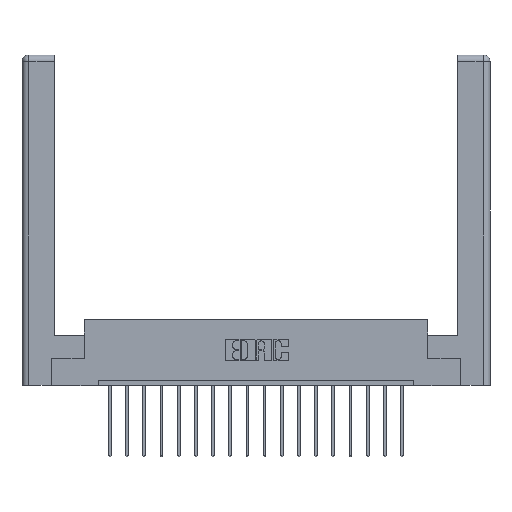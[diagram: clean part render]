
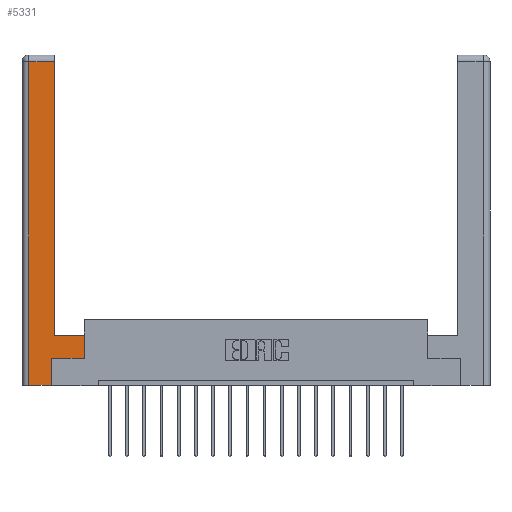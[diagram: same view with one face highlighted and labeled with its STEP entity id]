
A CAD part, top view. The second image highlights one B-rep face of the part: STEP entity #5331.
In plain terms, the highlighted planar face has unit normal (0, 0, 1).
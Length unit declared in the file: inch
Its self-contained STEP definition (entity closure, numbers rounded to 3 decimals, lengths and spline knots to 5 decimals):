
#281 = DIRECTION ( 'NONE',  ( 0., 1., 0. ) ) ;
#437 = CARTESIAN_POINT ( 'NONE',  ( 0.295, 0.45, 0. ) ) ;
#553 = VECTOR ( 'NONE', #10252, 39.37008 ) ;
#571 = LINE ( 'NONE', #16359, #12134 ) ;
#881 = CARTESIAN_POINT ( 'NONE',  ( 0.565, 0.45, 0. ) ) ;
#1206 = DIRECTION ( 'NONE',  ( -1., 0., 0. ) ) ;
#1996 = CARTESIAN_POINT ( 'NONE',  ( 0.565, 0.45, 0. ) ) ;
#2434 = CARTESIAN_POINT ( 'NONE',  ( 0.265, 0.245, 0. ) ) ;
#2443 = VECTOR ( 'NONE', #17867, 39.37008 ) ;
#2508 = EDGE_CURVE ( 'NONE', #7232, #6974, #3721, .T. ) ;
#2759 = VERTEX_POINT ( 'NONE', #10596 ) ;
#2766 = CARTESIAN_POINT ( 'NONE',  ( 0.265, 0.245, 0. ) ) ;
#3721 = LINE ( 'NONE', #8569, #12501 ) ;
#4185 = EDGE_CURVE ( 'NONE', #7661, #13098, #7813, .T. ) ;
#4265 = CARTESIAN_POINT ( 'NONE',  ( 0.265, 0., 0. ) ) ;
#5331 = ADVANCED_FACE ( 'NONE', ( #10559 ), #6381, .F. ) ;
#5668 = VERTEX_POINT ( 'NONE', #7271 ) ;
#5695 = EDGE_LOOP ( 'NONE', ( #7740, #14722, #8439, #8957, #5720, #6181, #9790, #7874 ) ) ;
#5720 = ORIENTED_EDGE ( 'NONE', *, *, #12259, .T. ) ;
#6181 = ORIENTED_EDGE ( 'NONE', *, *, #4185, .T. ) ;
#6354 = CARTESIAN_POINT ( 'NONE',  ( 0.565, 0.245, 0. ) ) ;
#6381 = PLANE ( 'NONE',  #6712 ) ;
#6584 = EDGE_CURVE ( 'NONE', #12918, #16740, #10551, .T. ) ;
#6712 = AXIS2_PLACEMENT_3D ( 'NONE', #10984, #16797, #13759 ) ;
#6974 = VERTEX_POINT ( 'NONE', #437 ) ;
#7118 = DIRECTION ( 'NONE',  ( 1., 0., 0. ) ) ;
#7232 = VERTEX_POINT ( 'NONE', #881 ) ;
#7271 = CARTESIAN_POINT ( 'NONE',  ( 0.295, 2.94, 0. ) ) ;
#7661 = VERTEX_POINT ( 'NONE', #2434 ) ;
#7740 = ORIENTED_EDGE ( 'NONE', *, *, #17522, .T. ) ;
#7813 = LINE ( 'NONE', #6354, #15218 ) ;
#7819 = VECTOR ( 'NONE', #281, 39.37008 ) ;
#7846 = DIRECTION ( 'NONE',  ( 1., 0., 0. ) ) ;
#7874 = ORIENTED_EDGE ( 'NONE', *, *, #2508, .T. ) ;
#8439 = ORIENTED_EDGE ( 'NONE', *, *, #6584, .T. ) ;
#8569 = CARTESIAN_POINT ( 'NONE',  ( 0.295, 0.45, 0. ) ) ;
#8861 = LINE ( 'NONE', #2766, #553 ) ;
#8957 = ORIENTED_EDGE ( 'NONE', *, *, #17435, .T. ) ;
#8976 = DIRECTION ( 'NONE',  ( 0., 1., 0. ) ) ;
#9052 = CARTESIAN_POINT ( 'NONE',  ( 0.0615, 0., 0. ) ) ;
#9705 = EDGE_CURVE ( 'NONE', #13098, #7232, #16158, .T. ) ;
#9790 = ORIENTED_EDGE ( 'NONE', *, *, #9705, .T. ) ;
#10252 = DIRECTION ( 'NONE',  ( 0., 1., 0. ) ) ;
#10344 = CARTESIAN_POINT ( 'NONE',  ( 0.0615, 2.94, 0. ) ) ;
#10551 = LINE ( 'NONE', #9052, #2443 ) ;
#10559 = FACE_OUTER_BOUND ( 'NONE', #5695, .T. ) ;
#10596 = CARTESIAN_POINT ( 'NONE',  ( 0.265, 0., 0. ) ) ;
#10984 = CARTESIAN_POINT ( 'NONE',  ( 0., 0., 0. ) ) ;
#11015 = CARTESIAN_POINT ( 'NONE',  ( 0.0615, 0., 0. ) ) ;
#11146 = VECTOR ( 'NONE', #7118, 39.37008 ) ;
#11862 = EDGE_CURVE ( 'NONE', #5668, #12918, #571, .T. ) ;
#12134 = VECTOR ( 'NONE', #17915, 39.37008 ) ;
#12259 = EDGE_CURVE ( 'NONE', #2759, #7661, #8861, .T. ) ;
#12501 = VECTOR ( 'NONE', #1206, 39.37008 ) ;
#12918 = VERTEX_POINT ( 'NONE', #10344 ) ;
#13003 = VECTOR ( 'NONE', #8976, 39.37008 ) ;
#13098 = VERTEX_POINT ( 'NONE', #16795 ) ;
#13388 = CARTESIAN_POINT ( 'NONE',  ( 0.295, 3., 0. ) ) ;
#13683 = LINE ( 'NONE', #13388, #13003 ) ;
#13759 = DIRECTION ( 'NONE',  ( -1., 0., 0. ) ) ;
#14722 = ORIENTED_EDGE ( 'NONE', *, *, #11862, .T. ) ;
#15218 = VECTOR ( 'NONE', #7846, 39.37008 ) ;
#16158 = LINE ( 'NONE', #1996, #7819 ) ;
#16359 = CARTESIAN_POINT ( 'NONE',  ( 0.0615, 2.94, 0. ) ) ;
#16740 = VERTEX_POINT ( 'NONE', #11015 ) ;
#16795 = CARTESIAN_POINT ( 'NONE',  ( 0.565, 0.245, 0. ) ) ;
#16797 = DIRECTION ( 'NONE',  ( 0., 0., -1. ) ) ;
#17401 = LINE ( 'NONE', #4265, #11146 ) ;
#17435 = EDGE_CURVE ( 'NONE', #16740, #2759, #17401, .T. ) ;
#17522 = EDGE_CURVE ( 'NONE', #6974, #5668, #13683, .T. ) ;
#17867 = DIRECTION ( 'NONE',  ( 0., -1., 0. ) ) ;
#17915 = DIRECTION ( 'NONE',  ( -1., 0., 0. ) ) ;
